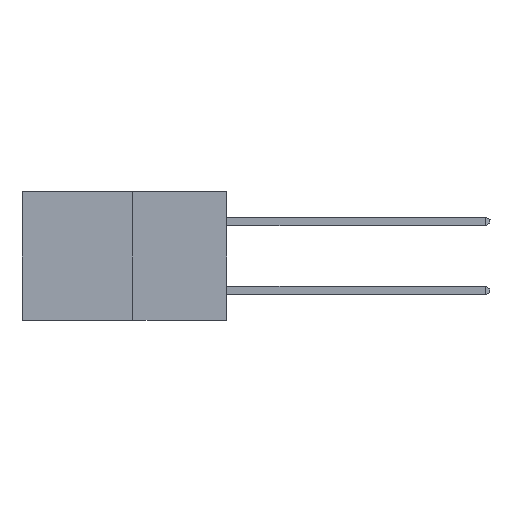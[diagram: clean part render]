
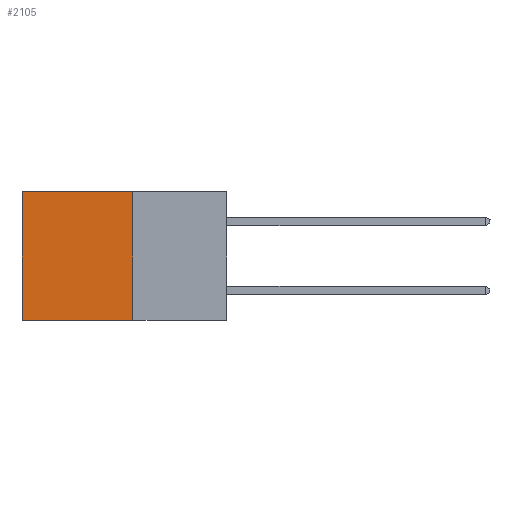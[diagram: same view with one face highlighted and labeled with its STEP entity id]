
A CAD part, left-side view. The second image highlights one B-rep face of the part: STEP entity #2105.
In plain terms, the highlighted planar face has unit normal (-1, 0, 0).
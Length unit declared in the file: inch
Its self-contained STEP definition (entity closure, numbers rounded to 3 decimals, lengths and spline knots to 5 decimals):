
#458 = EDGE_CURVE ( 'NONE', #21407, #13961, #11956, .T. ) ;
#1035 = DIRECTION ( 'NONE',  ( 0., 1., 0. ) ) ;
#1208 = CARTESIAN_POINT ( 'NONE',  ( 0.277, 0.27, 0. ) ) ;
#2105 = ADVANCED_FACE ( 'NONE', ( #3948 ), #4071, .F. ) ;
#2733 = CARTESIAN_POINT ( 'NONE',  ( 0.277, 0.27, -0.37 ) ) ;
#3723 = CARTESIAN_POINT ( 'NONE',  ( 0.277, 0.27, -0.37 ) ) ;
#3948 = FACE_OUTER_BOUND ( 'NONE', #17818, .T. ) ;
#4071 = PLANE ( 'NONE',  #11145 ) ;
#5127 = LINE ( 'NONE', #3723, #10293 ) ;
#5958 = VECTOR ( 'NONE', #1035, 39.37008 ) ;
#6315 = LINE ( 'NONE', #22433, #16089 ) ;
#7314 = DIRECTION ( 'NONE',  ( 0., 0., -1. ) ) ;
#7557 = VERTEX_POINT ( 'NONE', #21208 ) ;
#8206 = CARTESIAN_POINT ( 'NONE',  ( 0.277, 0.59, -0.37 ) ) ;
#9111 = EDGE_CURVE ( 'NONE', #18213, #21407, #16975, .T. ) ;
#10293 = VECTOR ( 'NONE', #19382, 39.37008 ) ;
#11145 = AXIS2_PLACEMENT_3D ( 'NONE', #2733, #20490, #7314 ) ;
#11956 = LINE ( 'NONE', #23798, #21188 ) ;
#12469 = EDGE_CURVE ( 'NONE', #7557, #13961, #5127, .T. ) ;
#12873 = EDGE_CURVE ( 'NONE', #18213, #7557, #6315, .T. ) ;
#13961 = VERTEX_POINT ( 'NONE', #8206 ) ;
#14292 = DIRECTION ( 'NONE',  ( 0., 0., -1. ) ) ;
#14514 = ORIENTED_EDGE ( 'NONE', *, *, #458, .T. ) ;
#15446 = ORIENTED_EDGE ( 'NONE', *, *, #12873, .F. ) ;
#16089 = VECTOR ( 'NONE', #24417, 39.37008 ) ;
#16975 = LINE ( 'NONE', #1208, #5958 ) ;
#17818 = EDGE_LOOP ( 'NONE', ( #14514, #24925, #15446, #24944 ) ) ;
#18213 = VERTEX_POINT ( 'NONE', #21102 ) ;
#19382 = DIRECTION ( 'NONE',  ( 0., 1., 0. ) ) ;
#20490 = DIRECTION ( 'NONE',  ( 1., 0., 0. ) ) ;
#21102 = CARTESIAN_POINT ( 'NONE',  ( 0.277, 0.27, 0. ) ) ;
#21188 = VECTOR ( 'NONE', #14292, 39.37008 ) ;
#21208 = CARTESIAN_POINT ( 'NONE',  ( 0.277, 0.27, -0.37 ) ) ;
#21407 = VERTEX_POINT ( 'NONE', #24274 ) ;
#22433 = CARTESIAN_POINT ( 'NONE',  ( 0.277, 0.27, -0.37 ) ) ;
#23798 = CARTESIAN_POINT ( 'NONE',  ( 0.277, 0.59, -0.37 ) ) ;
#24274 = CARTESIAN_POINT ( 'NONE',  ( 0.277, 0.59, 0. ) ) ;
#24417 = DIRECTION ( 'NONE',  ( 0., 0., -1. ) ) ;
#24925 = ORIENTED_EDGE ( 'NONE', *, *, #12469, .F. ) ;
#24944 = ORIENTED_EDGE ( 'NONE', *, *, #9111, .T. ) ;
